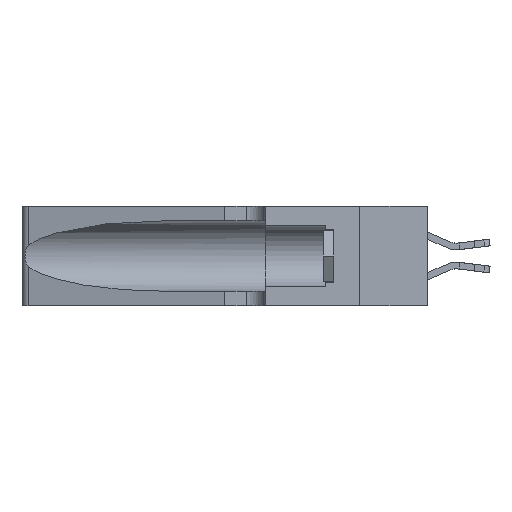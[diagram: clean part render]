
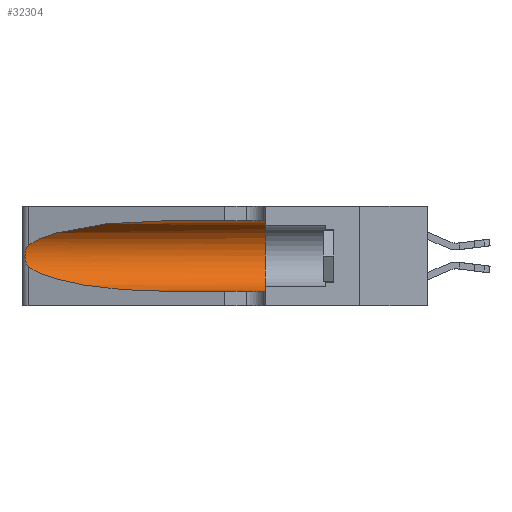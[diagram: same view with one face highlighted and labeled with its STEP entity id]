
A CAD part, left-side view. The second image highlights one B-rep face of the part: STEP entity #32304.
In plain terms, the highlighted cylindrical face has radius 3.308 mm (diameter 6.617 mm), a partial arc.
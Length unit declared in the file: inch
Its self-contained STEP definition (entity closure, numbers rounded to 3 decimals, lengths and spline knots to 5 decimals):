
#702 = VERTEX_POINT ( 'NONE', #20239 ) ;
#857 = ORIENTED_EDGE ( 'NONE', *, *, #32684, .T. ) ;
#891 = EDGE_CURVE ( 'NONE', #702, #17530, #3327, .T. ) ;
#2433 = CARTESIAN_POINT ( 'NONE',  ( 0.25787, 1.23484, 0.2124 ) ) ;
#2679 = CARTESIAN_POINT ( 'NONE',  ( 0.18966, 0.96281, 0.31525 ) ) ;
#3327 = LINE ( 'NONE', #12873, #9735 ) ;
#3649 = CYLINDRICAL_SURFACE ( 'NONE', #31743, 0.13025 ) ;
#4018 = VERTEX_POINT ( 'NONE', #27344 ) ;
#4328 = AXIS2_PLACEMENT_3D ( 'NONE', #16033, #34658, #18729 ) ;
#4849 = CARTESIAN_POINT ( 'NONE',  ( 0.25487, 1.22718, 0.22369 ) ) ;
#5152 = VERTEX_POINT ( 'NONE', #4849 ) ;
#5225 = CARTESIAN_POINT ( 'NONE',  ( 0.26018, 1.23835, 0.19895 ) ) ;
#5887 = CARTESIAN_POINT ( 'NONE',  ( 0.1305, 1.61858, 0.31525 ) ) ;
#6368 = B_SPLINE_CURVE_WITH_KNOTS ( 'NONE', 3,
 ( #13262, #29280, #18649, #2433, #21320, #5225, #24016, #7973, #26689, #10680, #29400, #13378, #32048, #16066 ),
 .UNSPECIFIED., .F., .F.,
 ( 4, 2, 2, 2, 2, 2, 4 ),
 ( 0., 0.00027, 0.00053, 0.00107, 0.0016, 0.00187, 0.00214 ),
 .UNSPECIFIED. ) ;
#6570 = CARTESIAN_POINT ( 'NONE',  ( 0.18966, 0.96281, 0.05475 ) ) ;
#6942 = ORIENTED_EDGE ( 'NONE', *, *, #891, .T. ) ;
#7444 =( BOUNDED_CURVE ( )  B_SPLINE_CURVE ( 3, ( #21574, #2679, #10923, #29634 ),
 .UNSPECIFIED., .F., .T. ) 
 B_SPLINE_CURVE_WITH_KNOTS ( ( 4, 4 ),
 ( 1.5708, 2.84003 ),
 .UNSPECIFIED. ) 
 CURVE ( )  GEOMETRIC_REPRESENTATION_ITEM ( )  RATIONAL_B_SPLINE_CURVE ( ( 1., 0.87, 0.87, 1. ) ) 
 REPRESENTATION_ITEM ( '' )  );
#7973 = CARTESIAN_POINT ( 'NONE',  ( 0.26075, 1.23896, 0.178 ) ) ;
#9735 = VECTOR ( 'NONE', #15550, 39.37008 ) ;
#10680 = CARTESIAN_POINT ( 'NONE',  ( 0.25856, 1.23593, 0.16098 ) ) ;
#10804 = EDGE_CURVE ( 'NONE', #23519, #18892, #19714, .T. ) ;
#10923 = CARTESIAN_POINT ( 'NONE',  ( 0.2373, 1.15595, 0.28018 ) ) ;
#12873 = CARTESIAN_POINT ( 'NONE',  ( 0.1305, 1.61858, 0.05475 ) ) ;
#13262 = CARTESIAN_POINT ( 'NONE',  ( 0.25487, 1.22718, 0.22369 ) ) ;
#13378 = CARTESIAN_POINT ( 'NONE',  ( 0.25639, 1.23186, 0.15144 ) ) ;
#13999 = ORIENTED_EDGE ( 'NONE', *, *, #10804, .F. ) ;
#14013 = DIRECTION ( 'NONE',  ( 0., -1., 0. ) ) ;
#14099 = ORIENTED_EDGE ( 'NONE', *, *, #27004, .T. ) ;
#14796 = DIRECTION ( 'NONE',  ( 0., -1., 0. ) ) ;
#15399 = EDGE_CURVE ( 'NONE', #5152, #4018, #6368, .T. ) ;
#15550 = DIRECTION ( 'NONE',  ( 0., -1., 0. ) ) ;
#16033 = CARTESIAN_POINT ( 'NONE',  ( 0.1305, 0.35, 0.185 ) ) ;
#16066 = CARTESIAN_POINT ( 'NONE',  ( 0.25487, 1.22718, 0.14631 ) ) ;
#17524 = DIRECTION ( 'NONE',  ( 0., 0., -1. ) ) ;
#17530 = VERTEX_POINT ( 'NONE', #29947 ) ;
#18649 = CARTESIAN_POINT ( 'NONE',  ( 0.25639, 1.23184, 0.21858 ) ) ;
#18729 = DIRECTION ( 'NONE',  ( 0., 0., 1. ) ) ;
#18880 = FACE_OUTER_BOUND ( 'NONE', #32087, .T. ) ;
#18892 = VERTEX_POINT ( 'NONE', #22119 ) ;
#19714 = LINE ( 'NONE', #5887, #33029 ) ;
#19941 = CARTESIAN_POINT ( 'NONE',  ( 0.2373, 1.15595, 0.08982 ) ) ;
#20239 = CARTESIAN_POINT ( 'NONE',  ( 0.1305, 0.72297, 0.05475 ) ) ;
#20854 = ORIENTED_EDGE ( 'NONE', *, *, #15399, .T. ) ;
#21320 = CARTESIAN_POINT ( 'NONE',  ( 0.25854, 1.2359, 0.20912 ) ) ;
#21574 = CARTESIAN_POINT ( 'NONE',  ( 0.1305, 0.72297, 0.31525 ) ) ;
#22119 = CARTESIAN_POINT ( 'NONE',  ( 0.1305, 0.35, 0.31525 ) ) ;
#23519 = VERTEX_POINT ( 'NONE', #33858 ) ;
#24016 = CARTESIAN_POINT ( 'NONE',  ( 0.26075, 1.23896, 0.19203 ) ) ;
#25328 = CARTESIAN_POINT ( 'NONE',  ( 0.1305, 0.72297, 0.05475 ) ) ;
#25450 = CARTESIAN_POINT ( 'NONE',  ( 0.1305, 1.61858, 0.185 ) ) ;
#26689 = CARTESIAN_POINT ( 'NONE',  ( 0.26017, 1.23833, 0.17102 ) ) ;
#27004 = EDGE_CURVE ( 'NONE', #4018, #702, #32307, .T. ) ;
#27344 = CARTESIAN_POINT ( 'NONE',  ( 0.25487, 1.22718, 0.14631 ) ) ;
#28796 = ORIENTED_EDGE ( 'NONE', *, *, #31387, .F. ) ;
#29280 = CARTESIAN_POINT ( 'NONE',  ( 0.25555, 1.22994, 0.2215 ) ) ;
#29400 = CARTESIAN_POINT ( 'NONE',  ( 0.25789, 1.23486, 0.15765 ) ) ;
#29634 = CARTESIAN_POINT ( 'NONE',  ( 0.25487, 1.22718, 0.22369 ) ) ;
#29947 = CARTESIAN_POINT ( 'NONE',  ( 0.1305, 0.35, 0.05475 ) ) ;
#31387 = EDGE_CURVE ( 'NONE', #18892, #17530, #33099, .T. ) ;
#31743 = AXIS2_PLACEMENT_3D ( 'NONE', #25450, #14796, #17524 ) ;
#32048 = CARTESIAN_POINT ( 'NONE',  ( 0.25555, 1.22993, 0.14849 ) ) ;
#32087 = EDGE_LOOP ( 'NONE', ( #857, #20854, #14099, #6942, #28796, #13999 ) ) ;
#32304 = ADVANCED_FACE ( 'NONE', ( #18880 ), #3649, .F. ) ;
#32307 =( BOUNDED_CURVE ( )  B_SPLINE_CURVE ( 3, ( #33220, #19941, #6570, #25328 ),
 .UNSPECIFIED., .F., .T. ) 
 B_SPLINE_CURVE_WITH_KNOTS ( ( 4, 4 ),
 ( 3.44316, 4.71239 ),
 .UNSPECIFIED. ) 
 CURVE ( )  GEOMETRIC_REPRESENTATION_ITEM ( )  RATIONAL_B_SPLINE_CURVE ( ( 1., 0.87, 0.87, 1. ) ) 
 REPRESENTATION_ITEM ( '' )  );
#32684 = EDGE_CURVE ( 'NONE', #23519, #5152, #7444, .T. ) ;
#33029 = VECTOR ( 'NONE', #14013, 39.37008 ) ;
#33099 = CIRCLE ( 'NONE', #4328, 0.13025 ) ;
#33220 = CARTESIAN_POINT ( 'NONE',  ( 0.25487, 1.22718, 0.14631 ) ) ;
#33858 = CARTESIAN_POINT ( 'NONE',  ( 0.1305, 0.72297, 0.31525 ) ) ;
#34658 = DIRECTION ( 'NONE',  ( 0., 1., 0. ) ) ;
